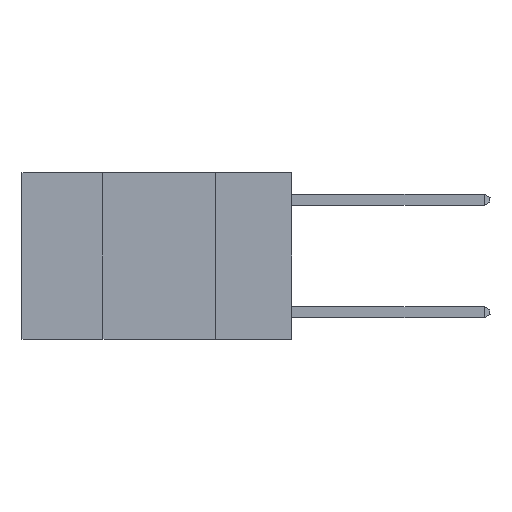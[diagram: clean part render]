
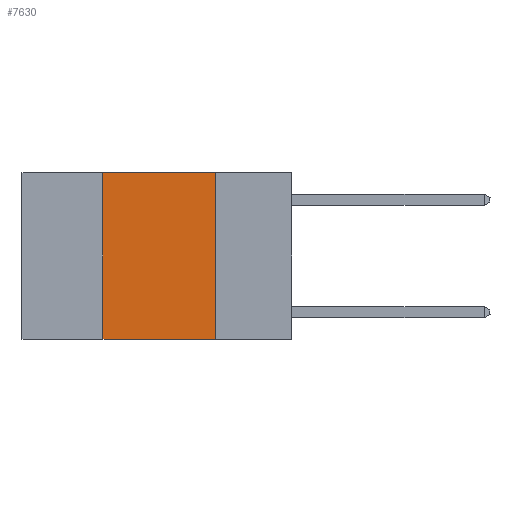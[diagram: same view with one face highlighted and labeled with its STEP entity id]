
A CAD part, left-side view. The second image highlights one B-rep face of the part: STEP entity #7630.
In plain terms, the highlighted planar face has unit normal (-1, 0, 0).
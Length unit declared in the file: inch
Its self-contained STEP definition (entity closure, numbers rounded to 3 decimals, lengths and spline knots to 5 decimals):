
#253 = VECTOR ( 'NONE', #3596, 39.37008 ) ;
#276 = CARTESIAN_POINT ( 'NONE',  ( 0., 0.42, -0.37 ) ) ;
#285 = DIRECTION ( 'NONE',  ( 0., 0., -1. ) ) ;
#373 = CARTESIAN_POINT ( 'NONE',  ( 0., 0.42, 0. ) ) ;
#806 = CARTESIAN_POINT ( 'NONE',  ( 0., 0.42, 0. ) ) ;
#1024 = DIRECTION ( 'NONE',  ( 0., -1., 0. ) ) ;
#1093 = PLANE ( 'NONE',  #4622 ) ;
#1171 = CARTESIAN_POINT ( 'NONE',  ( 0., 0.17, 0. ) ) ;
#1186 = ORIENTED_EDGE ( 'NONE', *, *, #1827, .F. ) ;
#1278 = LINE ( 'NONE', #1171, #7981 ) ;
#1463 = VERTEX_POINT ( 'NONE', #4545 ) ;
#1827 = EDGE_CURVE ( 'NONE', #8067, #2084, #7590, .T. ) ;
#1982 = ORIENTED_EDGE ( 'NONE', *, *, #3009, .F. ) ;
#2062 = VERTEX_POINT ( 'NONE', #2331 ) ;
#2084 = VERTEX_POINT ( 'NONE', #806 ) ;
#2331 = CARTESIAN_POINT ( 'NONE',  ( 0., 0.17, -0.37 ) ) ;
#3009 = EDGE_CURVE ( 'NONE', #2084, #1463, #3721, .T. ) ;
#3214 = ORIENTED_EDGE ( 'NONE', *, *, #9237, .T. ) ;
#3596 = DIRECTION ( 'NONE',  ( 0., 0., 1. ) ) ;
#3721 = LINE ( 'NONE', #6836, #8428 ) ;
#4183 = LINE ( 'NONE', #7385, #4975 ) ;
#4301 = CARTESIAN_POINT ( 'NONE',  ( 0., 0.6, 0. ) ) ;
#4545 = CARTESIAN_POINT ( 'NONE',  ( 0., 0.17, 0. ) ) ;
#4622 = AXIS2_PLACEMENT_3D ( 'NONE', #4301, #7499, #285 ) ;
#4975 = VECTOR ( 'NONE', #1024, 39.37008 ) ;
#5076 = FACE_OUTER_BOUND ( 'NONE', #5719, .T. ) ;
#5215 = DIRECTION ( 'NONE',  ( 0., 0., -1. ) ) ;
#5312 = DIRECTION ( 'NONE',  ( 0., -1., 0. ) ) ;
#5719 = EDGE_LOOP ( 'NONE', ( #7874, #1982, #1186, #3214 ) ) ;
#5774 = EDGE_CURVE ( 'NONE', #1463, #2062, #1278, .T. ) ;
#6836 = CARTESIAN_POINT ( 'NONE',  ( 0., 0.6, 0. ) ) ;
#7385 = CARTESIAN_POINT ( 'NONE',  ( 0., 0.6, -0.37 ) ) ;
#7499 = DIRECTION ( 'NONE',  ( 1., 0., 0. ) ) ;
#7590 = LINE ( 'NONE', #373, #253 ) ;
#7630 = ADVANCED_FACE ( 'NONE', ( #5076 ), #1093, .F. ) ;
#7874 = ORIENTED_EDGE ( 'NONE', *, *, #5774, .F. ) ;
#7981 = VECTOR ( 'NONE', #5215, 39.37008 ) ;
#8067 = VERTEX_POINT ( 'NONE', #276 ) ;
#8428 = VECTOR ( 'NONE', #5312, 39.37008 ) ;
#9237 = EDGE_CURVE ( 'NONE', #8067, #2062, #4183, .T. ) ;
